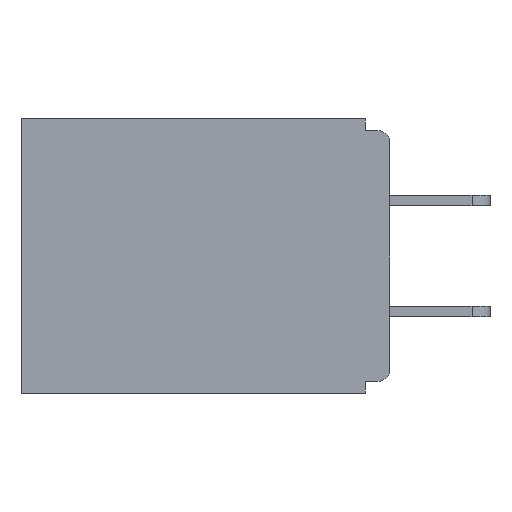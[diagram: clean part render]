
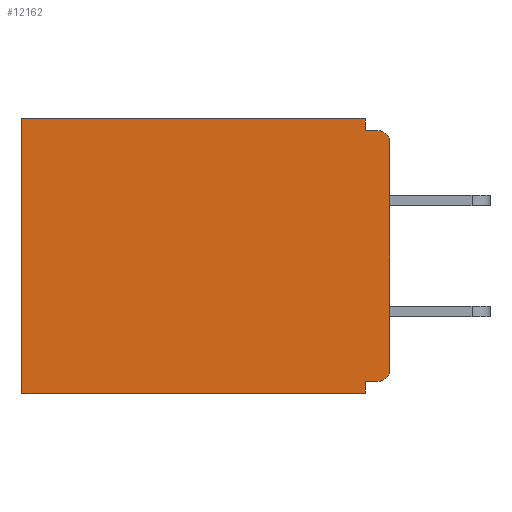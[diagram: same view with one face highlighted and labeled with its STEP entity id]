
A CAD part, left-side view. The second image highlights one B-rep face of the part: STEP entity #12162.
In plain terms, the highlighted planar face has unit normal (-1, 0, 0).
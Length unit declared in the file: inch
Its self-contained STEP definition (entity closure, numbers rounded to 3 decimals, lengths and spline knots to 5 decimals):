
#627 = VERTEX_POINT ( 'NONE', #9095 ) ;
#896 = CARTESIAN_POINT ( 'NONE',  ( 0.298, 0.46, 0. ) ) ;
#1011 = ORIENTED_EDGE ( 'NONE', *, *, #2555, .F. ) ;
#1308 = CARTESIAN_POINT ( 'NONE',  ( 0.298, 0.015, -0.313 ) ) ;
#1368 = EDGE_CURVE ( 'NONE', #7289, #4067, #5098, .T. ) ;
#1692 = DIRECTION ( 'NONE',  ( 0., 0., -1. ) ) ;
#1806 = CARTESIAN_POINT ( 'NONE',  ( 0.298, 0.015, -0.015 ) ) ;
#1823 = CARTESIAN_POINT ( 'NONE',  ( 0.298, 0., -0.328 ) ) ;
#2175 = LINE ( 'NONE', #5943, #7611 ) ;
#2213 = DIRECTION ( 'NONE',  ( 0., 0., -1. ) ) ;
#2267 = VERTEX_POINT ( 'NONE', #5779 ) ;
#2324 = CARTESIAN_POINT ( 'NONE',  ( 0.298, 0.031, -0.343 ) ) ;
#2328 = CARTESIAN_POINT ( 'NONE',  ( 0.298, 0.031, -0.343 ) ) ;
#2373 = ORIENTED_EDGE ( 'NONE', *, *, #7730, .F. ) ;
#2472 = CARTESIAN_POINT ( 'NONE',  ( 0.298, 0., -0.03 ) ) ;
#2555 = EDGE_CURVE ( 'NONE', #10122, #3782, #8504, .T. ) ;
#2612 = DIRECTION ( 'NONE',  ( 1., 0., 0. ) ) ;
#2693 = CARTESIAN_POINT ( 'NONE',  ( 0.298, 0.031, 0. ) ) ;
#3004 = AXIS2_PLACEMENT_3D ( 'NONE', #4681, #2612, #6780 ) ;
#3095 = DIRECTION ( 'NONE',  ( -1., 0., 0. ) ) ;
#3614 = DIRECTION ( 'NONE',  ( 0., 1., 0. ) ) ;
#3782 = VERTEX_POINT ( 'NONE', #5109 ) ;
#3964 = VERTEX_POINT ( 'NONE', #896 ) ;
#4067 = VERTEX_POINT ( 'NONE', #2328 ) ;
#4401 = DIRECTION ( 'NONE',  ( 0., 0., -1. ) ) ;
#4410 = LINE ( 'NONE', #1823, #9766 ) ;
#4411 = EDGE_CURVE ( 'NONE', #10122, #3964, #2175, .T. ) ;
#4567 = DIRECTION ( 'NONE',  ( 0., 1., 0. ) ) ;
#4681 = CARTESIAN_POINT ( 'NONE',  ( 0.298, 0., 0. ) ) ;
#4698 = VERTEX_POINT ( 'NONE', #2472 ) ;
#4721 = EDGE_CURVE ( 'NONE', #4067, #627, #6969, .T. ) ;
#4752 = FACE_OUTER_BOUND ( 'NONE', #8718, .T. ) ;
#5006 = ORIENTED_EDGE ( 'NONE', *, *, #1368, .F. ) ;
#5098 = LINE ( 'NONE', #2324, #11658 ) ;
#5109 = CARTESIAN_POINT ( 'NONE',  ( 0.298, 0.031, -0.015 ) ) ;
#5298 = DIRECTION ( 'NONE',  ( 0., 0., -1. ) ) ;
#5599 = EDGE_CURVE ( 'NONE', #9973, #7289, #4410, .T. ) ;
#5779 = CARTESIAN_POINT ( 'NONE',  ( 0.298, 0., -0.313 ) ) ;
#5903 = ORIENTED_EDGE ( 'NONE', *, *, #4721, .F. ) ;
#5943 = CARTESIAN_POINT ( 'NONE',  ( 0.298, 0., 0. ) ) ;
#6588 = ORIENTED_EDGE ( 'NONE', *, *, #9537, .T. ) ;
#6592 = CARTESIAN_POINT ( 'NONE',  ( 0.298, 0.031, -0.343 ) ) ;
#6780 = DIRECTION ( 'NONE',  ( 0., 0., -1. ) ) ;
#6831 = DIRECTION ( 'NONE',  ( 0., 0., -1. ) ) ;
#6843 = ORIENTED_EDGE ( 'NONE', *, *, #4411, .T. ) ;
#6969 = LINE ( 'NONE', #11195, #10675 ) ;
#7037 = DIRECTION ( 'NONE',  ( 0., 1., 0. ) ) ;
#7222 = EDGE_CURVE ( 'NONE', #3782, #10568, #7901, .T. ) ;
#7289 = VERTEX_POINT ( 'NONE', #11412 ) ;
#7295 = ORIENTED_EDGE ( 'NONE', *, *, #8874, .T. ) ;
#7400 = CARTESIAN_POINT ( 'NONE',  ( 0.298, 0., -0.015 ) ) ;
#7611 = VECTOR ( 'NONE', #7037, 39.37008 ) ;
#7669 = ORIENTED_EDGE ( 'NONE', *, *, #5599, .F. ) ;
#7730 = EDGE_CURVE ( 'NONE', #4698, #2267, #7739, .T. ) ;
#7737 = ORIENTED_EDGE ( 'NONE', *, *, #9216, .T. ) ;
#7739 = LINE ( 'NONE', #10185, #9631 ) ;
#7901 = LINE ( 'NONE', #7400, #10390 ) ;
#8009 = LINE ( 'NONE', #9198, #8446 ) ;
#8286 = CIRCLE ( 'NONE', #10252, 0.015 ) ;
#8296 = CIRCLE ( 'NONE', #11130, 0.015 ) ;
#8446 = VECTOR ( 'NONE', #2213, 39.37008 ) ;
#8470 = DIRECTION ( 'NONE',  ( 0., -1., 0. ) ) ;
#8504 = LINE ( 'NONE', #6592, #10270 ) ;
#8718 = EDGE_LOOP ( 'NONE', ( #6588, #10463, #1011, #6843, #7295, #5903, #5006, #7669, #7737, #2373 ) ) ;
#8736 = CARTESIAN_POINT ( 'NONE',  ( 0.298, 0.015, -0.03 ) ) ;
#8874 = EDGE_CURVE ( 'NONE', #3964, #627, #8009, .T. ) ;
#9018 = DIRECTION ( 'NONE',  ( 0., 0., -1. ) ) ;
#9095 = CARTESIAN_POINT ( 'NONE',  ( 0.298, 0.46, -0.343 ) ) ;
#9198 = CARTESIAN_POINT ( 'NONE',  ( 0.298, 0.46, 0. ) ) ;
#9216 = EDGE_CURVE ( 'NONE', #9973, #2267, #8296, .T. ) ;
#9537 = EDGE_CURVE ( 'NONE', #4698, #10568, #8286, .T. ) ;
#9631 = VECTOR ( 'NONE', #1692, 39.37008 ) ;
#9766 = VECTOR ( 'NONE', #4567, 39.37008 ) ;
#9973 = VERTEX_POINT ( 'NONE', #12104 ) ;
#10122 = VERTEX_POINT ( 'NONE', #2693 ) ;
#10185 = CARTESIAN_POINT ( 'NONE',  ( 0.298, 0., 0. ) ) ;
#10252 = AXIS2_PLACEMENT_3D ( 'NONE', #8736, #3095, #6831 ) ;
#10270 = VECTOR ( 'NONE', #4401, 39.37008 ) ;
#10374 = PLANE ( 'NONE',  #3004 ) ;
#10390 = VECTOR ( 'NONE', #8470, 39.37008 ) ;
#10463 = ORIENTED_EDGE ( 'NONE', *, *, #7222, .F. ) ;
#10568 = VERTEX_POINT ( 'NONE', #1806 ) ;
#10675 = VECTOR ( 'NONE', #3614, 39.37008 ) ;
#11130 = AXIS2_PLACEMENT_3D ( 'NONE', #1308, #11948, #5298 ) ;
#11195 = CARTESIAN_POINT ( 'NONE',  ( 0.298, 0., -0.343 ) ) ;
#11412 = CARTESIAN_POINT ( 'NONE',  ( 0.298, 0.031, -0.328 ) ) ;
#11658 = VECTOR ( 'NONE', #9018, 39.37008 ) ;
#11948 = DIRECTION ( 'NONE',  ( -1., 0., 0. ) ) ;
#12104 = CARTESIAN_POINT ( 'NONE',  ( 0.298, 0.015, -0.328 ) ) ;
#12162 = ADVANCED_FACE ( 'NONE', ( #4752 ), #10374, .F. ) ;
